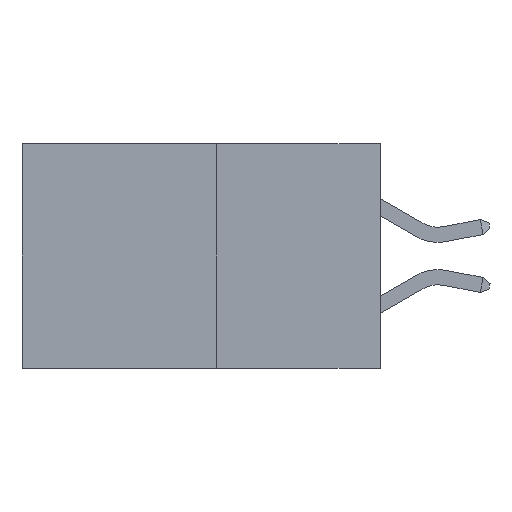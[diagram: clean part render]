
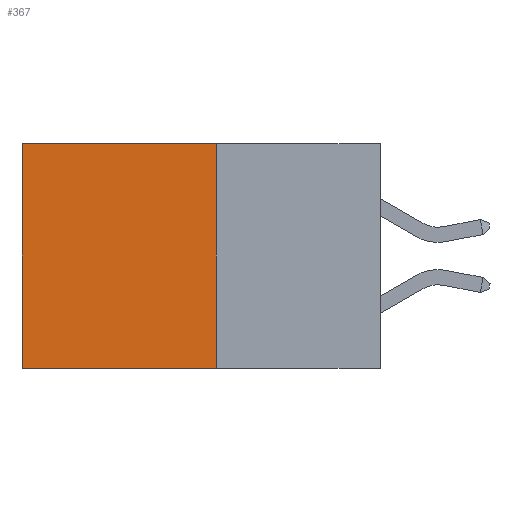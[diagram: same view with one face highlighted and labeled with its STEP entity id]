
A CAD part, left-side view. The second image highlights one B-rep face of the part: STEP entity #367.
In plain terms, the highlighted planar face has unit normal (-1, 0, 0).
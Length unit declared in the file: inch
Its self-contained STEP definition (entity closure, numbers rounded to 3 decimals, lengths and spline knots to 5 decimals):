
#34 = DIRECTION ( 'NONE',  ( 1., 0., 0. ) ) ;
#367 = ADVANCED_FACE ( 'NONE', ( #3501 ), #6635, .F. ) ;
#550 = DIRECTION ( 'NONE',  ( 0., 1., 0. ) ) ;
#761 = EDGE_CURVE ( 'NONE', #12846, #3191, #13036, .T. ) ;
#2020 = AXIS2_PLACEMENT_3D ( 'NONE', #17842, #34, #3914 ) ;
#2111 = VECTOR ( 'NONE', #3017, 39.37008 ) ;
#2663 = CARTESIAN_POINT ( 'NONE',  ( 0.277, 0.27, 0. ) ) ;
#2938 = VERTEX_POINT ( 'NONE', #2663 ) ;
#3017 = DIRECTION ( 'NONE',  ( 0., 0., -1. ) ) ;
#3191 = VERTEX_POINT ( 'NONE', #19259 ) ;
#3501 = FACE_OUTER_BOUND ( 'NONE', #9895, .T. ) ;
#3914 = DIRECTION ( 'NONE',  ( 0., 0., -1. ) ) ;
#4150 = CARTESIAN_POINT ( 'NONE',  ( 0.277, 0.59, 0. ) ) ;
#4324 = VECTOR ( 'NONE', #19103, 39.37008 ) ;
#5660 = EDGE_CURVE ( 'NONE', #2938, #15043, #10047, .T. ) ;
#6165 = LINE ( 'NONE', #8680, #2111 ) ;
#6635 = PLANE ( 'NONE',  #2020 ) ;
#7096 = CARTESIAN_POINT ( 'NONE',  ( 0.277, 0.27, -0.37 ) ) ;
#8680 = CARTESIAN_POINT ( 'NONE',  ( 0.277, 0.59, -0.37 ) ) ;
#9895 = EDGE_LOOP ( 'NONE', ( #11829, #10512, #12348, #16631 ) ) ;
#10047 = LINE ( 'NONE', #13848, #14123 ) ;
#10512 = ORIENTED_EDGE ( 'NONE', *, *, #761, .F. ) ;
#11829 = ORIENTED_EDGE ( 'NONE', *, *, #13468, .T. ) ;
#12348 = ORIENTED_EDGE ( 'NONE', *, *, #16333, .F. ) ;
#12846 = VERTEX_POINT ( 'NONE', #13880 ) ;
#13036 = LINE ( 'NONE', #7096, #16029 ) ;
#13468 = EDGE_CURVE ( 'NONE', #15043, #3191, #6165, .T. ) ;
#13848 = CARTESIAN_POINT ( 'NONE',  ( 0.277, 0.27, 0. ) ) ;
#13850 = DIRECTION ( 'NONE',  ( 0., 1., 0. ) ) ;
#13880 = CARTESIAN_POINT ( 'NONE',  ( 0.277, 0.27, -0.37 ) ) ;
#14123 = VECTOR ( 'NONE', #13850, 39.37008 ) ;
#15043 = VERTEX_POINT ( 'NONE', #4150 ) ;
#16029 = VECTOR ( 'NONE', #550, 39.37008 ) ;
#16333 = EDGE_CURVE ( 'NONE', #2938, #12846, #16386, .T. ) ;
#16386 = LINE ( 'NONE', #17582, #4324 ) ;
#16631 = ORIENTED_EDGE ( 'NONE', *, *, #5660, .T. ) ;
#17582 = CARTESIAN_POINT ( 'NONE',  ( 0.277, 0.27, -0.37 ) ) ;
#17842 = CARTESIAN_POINT ( 'NONE',  ( 0.277, 0.27, -0.37 ) ) ;
#19103 = DIRECTION ( 'NONE',  ( 0., 0., -1. ) ) ;
#19259 = CARTESIAN_POINT ( 'NONE',  ( 0.277, 0.59, -0.37 ) ) ;
